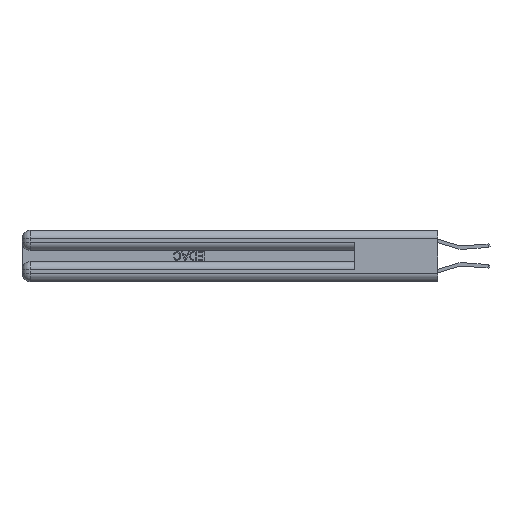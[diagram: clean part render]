
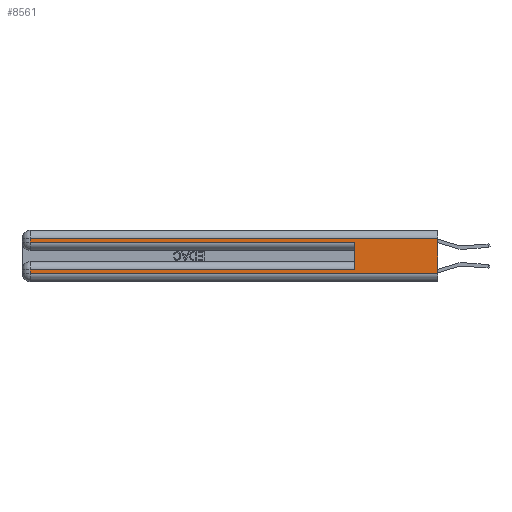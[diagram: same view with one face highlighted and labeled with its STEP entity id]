
A CAD part, left-side view. The second image highlights one B-rep face of the part: STEP entity #8561.
In plain terms, the highlighted planar face has unit normal (-1, 0, 0).
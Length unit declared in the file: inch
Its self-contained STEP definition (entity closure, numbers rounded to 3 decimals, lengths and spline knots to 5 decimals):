
#137 = LINE ( 'NONE', #30080, #14391 ) ;
#1323 = CARTESIAN_POINT ( 'NONE',  ( 0., 0.6, 0.285 ) ) ;
#1547 = ORIENTED_EDGE ( 'NONE', *, *, #30156, .F. ) ;
#2406 = EDGE_CURVE ( 'NONE', #28484, #20315, #35533, .T. ) ;
#2645 = DIRECTION ( 'NONE',  ( 1., 0., 0. ) ) ;
#2882 = VERTEX_POINT ( 'NONE', #29793 ) ;
#4480 = VECTOR ( 'NONE', #9702, 39.37008 ) ;
#4551 = EDGE_CURVE ( 'NONE', #17862, #12502, #137, .T. ) ;
#5463 = CARTESIAN_POINT ( 'NONE',  ( 0., 2.94, 0.31 ) ) ;
#6192 = EDGE_LOOP ( 'NONE', ( #1547, #24435, #30426, #14008, #28919, #23607, #25099, #16683 ) ) ;
#6331 = EDGE_CURVE ( 'NONE', #7464, #9412, #7175, .T. ) ;
#6913 = DIRECTION ( 'NONE',  ( 0., 0., -1. ) ) ;
#7175 = LINE ( 'NONE', #11099, #4480 ) ;
#7464 = VERTEX_POINT ( 'NONE', #8670 ) ;
#7527 = VECTOR ( 'NONE', #13616, 39.37008 ) ;
#8561 = ADVANCED_FACE ( 'NONE', ( #28890 ), #14221, .F. ) ;
#8670 = CARTESIAN_POINT ( 'NONE',  ( 0., 2.94, 0.285 ) ) ;
#9412 = VERTEX_POINT ( 'NONE', #1323 ) ;
#9445 = CARTESIAN_POINT ( 'NONE',  ( 0., 2.94, 0.085 ) ) ;
#9702 = DIRECTION ( 'NONE',  ( 0., -1., 0. ) ) ;
#10436 = CARTESIAN_POINT ( 'NONE',  ( 0., 0.6, 0.145 ) ) ;
#10748 = CARTESIAN_POINT ( 'NONE',  ( 0., 2.94, 0.37 ) ) ;
#11099 = CARTESIAN_POINT ( 'NONE',  ( 0., 0., 0.285 ) ) ;
#11830 = CARTESIAN_POINT ( 'NONE',  ( 0., 0., 0.37 ) ) ;
#12502 = VERTEX_POINT ( 'NONE', #5463 ) ;
#13021 = EDGE_CURVE ( 'NONE', #2882, #9412, #35778, .T. ) ;
#13616 = DIRECTION ( 'NONE',  ( 0., 0., -1. ) ) ;
#13707 = VECTOR ( 'NONE', #35398, 39.37008 ) ;
#14008 = ORIENTED_EDGE ( 'NONE', *, *, #6331, .T. ) ;
#14221 = PLANE ( 'NONE',  #20766 ) ;
#14340 = DIRECTION ( 'NONE',  ( 0., 0., -1. ) ) ;
#14391 = VECTOR ( 'NONE', #28330, 39.37008 ) ;
#14541 = LINE ( 'NONE', #11830, #18971 ) ;
#14601 = DIRECTION ( 'NONE',  ( 0., -1., 0. ) ) ;
#14617 = CARTESIAN_POINT ( 'NONE',  ( 0., 0., 0.085 ) ) ;
#14941 = CARTESIAN_POINT ( 'NONE',  ( 0., 0., 0.06 ) ) ;
#15013 = LINE ( 'NONE', #14617, #13707 ) ;
#15100 = LINE ( 'NONE', #10748, #7527 ) ;
#15396 = CARTESIAN_POINT ( 'NONE',  ( 0., 2.94, 0.37 ) ) ;
#15746 = VECTOR ( 'NONE', #27726, 39.37008 ) ;
#16620 = EDGE_CURVE ( 'NONE', #2882, #28484, #15013, .T. ) ;
#16683 = ORIENTED_EDGE ( 'NONE', *, *, #30870, .T. ) ;
#17862 = VERTEX_POINT ( 'NONE', #30112 ) ;
#18971 = VECTOR ( 'NONE', #14340, 39.37008 ) ;
#20315 = VERTEX_POINT ( 'NONE', #27651 ) ;
#20766 = AXIS2_PLACEMENT_3D ( 'NONE', #28523, #2645, #22562 ) ;
#21638 = EDGE_CURVE ( 'NONE', #12502, #7464, #15100, .T. ) ;
#22096 = VERTEX_POINT ( 'NONE', #14941 ) ;
#22562 = DIRECTION ( 'NONE',  ( 0., 0., -1. ) ) ;
#23607 = ORIENTED_EDGE ( 'NONE', *, *, #16620, .T. ) ;
#24435 = ORIENTED_EDGE ( 'NONE', *, *, #4551, .T. ) ;
#25099 = ORIENTED_EDGE ( 'NONE', *, *, #2406, .T. ) ;
#27651 = CARTESIAN_POINT ( 'NONE',  ( 0., 2.94, 0.06 ) ) ;
#27726 = DIRECTION ( 'NONE',  ( 0., 0., 1. ) ) ;
#27958 = VECTOR ( 'NONE', #6913, 39.37008 ) ;
#28330 = DIRECTION ( 'NONE',  ( 0., 1., 0. ) ) ;
#28484 = VERTEX_POINT ( 'NONE', #9445 ) ;
#28523 = CARTESIAN_POINT ( 'NONE',  ( 0., 0., 0.37 ) ) ;
#28890 = FACE_OUTER_BOUND ( 'NONE', #6192, .T. ) ;
#28919 = ORIENTED_EDGE ( 'NONE', *, *, #13021, .F. ) ;
#29793 = CARTESIAN_POINT ( 'NONE',  ( 0., 0.6, 0.085 ) ) ;
#30080 = CARTESIAN_POINT ( 'NONE',  ( 0., 0., 0.31 ) ) ;
#30112 = CARTESIAN_POINT ( 'NONE',  ( 0., 0., 0.31 ) ) ;
#30156 = EDGE_CURVE ( 'NONE', #17862, #22096, #14541, .T. ) ;
#30426 = ORIENTED_EDGE ( 'NONE', *, *, #21638, .T. ) ;
#30870 = EDGE_CURVE ( 'NONE', #20315, #22096, #30988, .T. ) ;
#30988 = LINE ( 'NONE', #31774, #35866 ) ;
#31774 = CARTESIAN_POINT ( 'NONE',  ( 0., 0., 0.06 ) ) ;
#35398 = DIRECTION ( 'NONE',  ( 0., 1., 0. ) ) ;
#35533 = LINE ( 'NONE', #15396, #27958 ) ;
#35778 = LINE ( 'NONE', #10436, #15746 ) ;
#35866 = VECTOR ( 'NONE', #14601, 39.37008 ) ;
